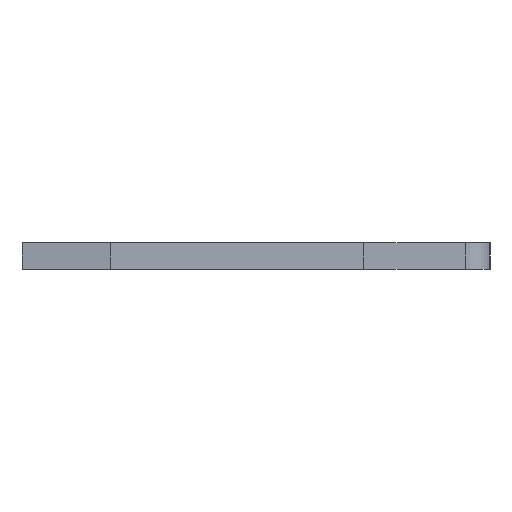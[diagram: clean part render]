
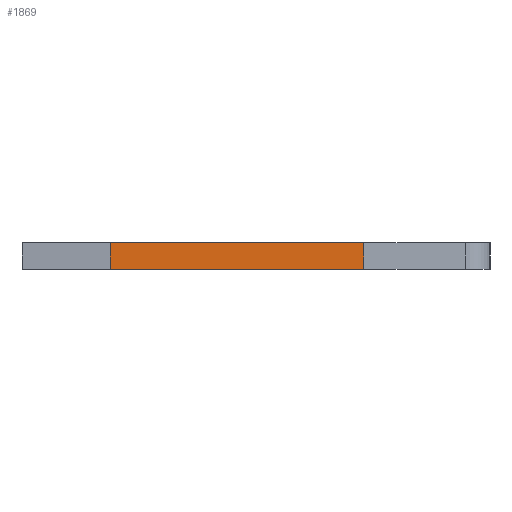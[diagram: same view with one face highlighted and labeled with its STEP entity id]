
A CAD part, left-side view. The second image highlights one B-rep face of the part: STEP entity #1869.
In plain terms, the highlighted face is planar.
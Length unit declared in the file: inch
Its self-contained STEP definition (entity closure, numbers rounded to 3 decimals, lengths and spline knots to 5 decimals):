
#76 = FACE_OUTER_BOUND ( 'NONE', #260, .T. ) ;
#202 = LINE ( 'NONE', #598, #2091 ) ;
#250 = LINE ( 'NONE', #1841, #1092 ) ;
#260 = EDGE_LOOP ( 'NONE', ( #303, #1163, #1239, #496 ) ) ;
#303 = ORIENTED_EDGE ( 'NONE', *, *, #1262, .T. ) ;
#326 = VERTEX_POINT ( 'NONE', #392 ) ;
#341 = VERTEX_POINT ( 'NONE', #1236 ) ;
#392 = CARTESIAN_POINT ( 'NONE',  ( -0.013, 0.146, -0.0575 ) ) ;
#496 = ORIENTED_EDGE ( 'NONE', *, *, #1152, .T. ) ;
#567 = DIRECTION ( 'NONE',  ( 0., 0., 1. ) ) ;
#598 = CARTESIAN_POINT ( 'NONE',  ( 0.013, 0.146, -0.0575 ) ) ;
#811 = EDGE_CURVE ( 'NONE', #1802, #1875, #202, .T. ) ;
#882 = LINE ( 'NONE', #1242, #1715 ) ;
#893 = CARTESIAN_POINT ( 'NONE',  ( 0.013, 0.146, -0.0575 ) ) ;
#1001 = CARTESIAN_POINT ( 'NONE',  ( -0.013, 0.146, -0.0575 ) ) ;
#1008 = DIRECTION ( 'NONE',  ( 0., 1., 0. ) ) ;
#1084 = PLANE ( 'NONE',  #1414 ) ;
#1092 = VECTOR ( 'NONE', #1153, 39.37008 ) ;
#1152 = EDGE_CURVE ( 'NONE', #1802, #341, #250, .T. ) ;
#1153 = DIRECTION ( 'NONE',  ( -1., 0., 0. ) ) ;
#1163 = ORIENTED_EDGE ( 'NONE', *, *, #1858, .F. ) ;
#1236 = CARTESIAN_POINT ( 'NONE',  ( -0.013, -0.099, -0.0575 ) ) ;
#1239 = ORIENTED_EDGE ( 'NONE', *, *, #811, .F. ) ;
#1242 = CARTESIAN_POINT ( 'NONE',  ( 0.013, 0.146, -0.0575 ) ) ;
#1262 = EDGE_CURVE ( 'NONE', #341, #326, #1509, .T. ) ;
#1328 = VECTOR ( 'NONE', #1008, 39.37008 ) ;
#1411 = CARTESIAN_POINT ( 'NONE',  ( 0.013, -0.099, -0.0575 ) ) ;
#1414 = AXIS2_PLACEMENT_3D ( 'NONE', #893, #567, #1727 ) ;
#1439 = DIRECTION ( 'NONE',  ( 0., 1., 0. ) ) ;
#1509 = LINE ( 'NONE', #1001, #1328 ) ;
#1559 = CARTESIAN_POINT ( 'NONE',  ( 0.013, 0.146, -0.0575 ) ) ;
#1715 = VECTOR ( 'NONE', #1747, 39.37008 ) ;
#1727 = DIRECTION ( 'NONE',  ( 1., 0., 0. ) ) ;
#1747 = DIRECTION ( 'NONE',  ( -1., 0., 0. ) ) ;
#1802 = VERTEX_POINT ( 'NONE', #1411 ) ;
#1841 = CARTESIAN_POINT ( 'NONE',  ( 0.013, -0.099, -0.0575 ) ) ;
#1858 = EDGE_CURVE ( 'NONE', #1875, #326, #882, .T. ) ;
#1869 = ADVANCED_FACE ( 'NONE', ( #76 ), #1084, .F. ) ;
#1875 = VERTEX_POINT ( 'NONE', #1559 ) ;
#2091 = VECTOR ( 'NONE', #1439, 39.37008 ) ;
